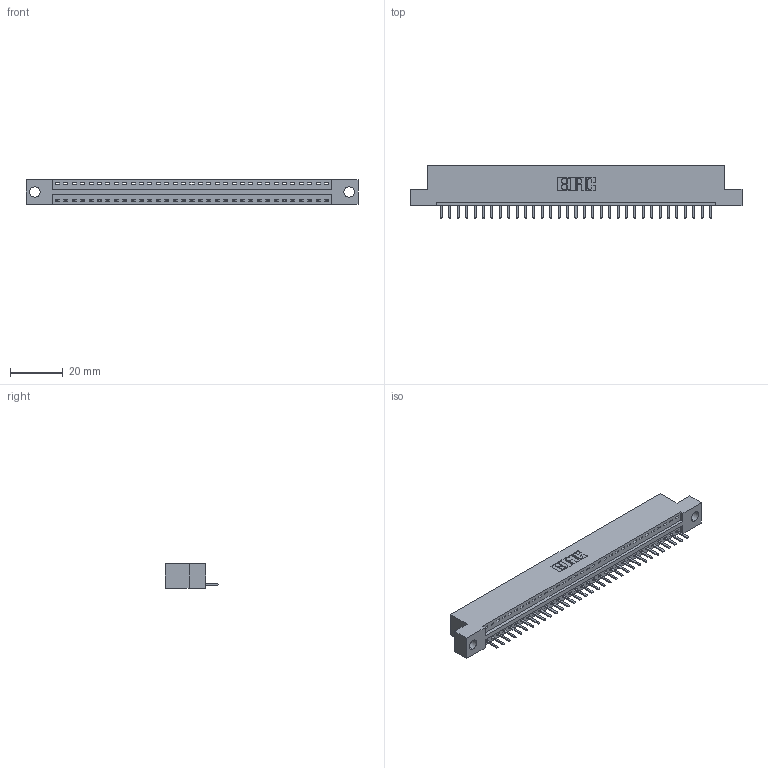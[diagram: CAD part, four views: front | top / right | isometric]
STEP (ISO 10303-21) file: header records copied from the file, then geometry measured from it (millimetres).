
FILE_DESCRIPTION (( 'STEP AP203' ), '1' );
FILE_NAME ('346-033-520-104.STEP', '2022-05-06T19:16:41', ( '' ), ( '' ), 'SwSTEP 2.0', 'SolidWorks 2020', '' );
FILE_SCHEMA (( 'CONFIG_CONTROL_DESIGN' ));
Length unit declared in the file: inch
Products named in the file (3): 345-292-001_345-293-120; 346-033-520-104; 346 Part_Flush Mounting Lugs - 0.156 Dia-TH
Assembly tree (34 placements, depth 2):
  346-033-520-104
    346 Part_Flush Mounting Lugs - 0.156 Dia-TH
    345-292-001_345-293-120  x33
Bounding box: 125.35 x 20.02 x 9.4 mm (x, y, z)
Volume: 11735.8 mm3; surface area: 14091.5 mm2
Topology: 34 solids, 34 shells, 2182 faces, 6437 edges, 4202 vertices
Faces by surface type: plane 1476, cylinder 706
Entity records: 22225 total; most frequent: CARTESIAN_POINT 3833, ORIENTED_EDGE 3786, DIRECTION 3379, EDGE_CURVE 1893, LINE 1625, VECTOR 1625, VERTEX_POINT 1258, AXIS2_PLACEMENT_3D 877
